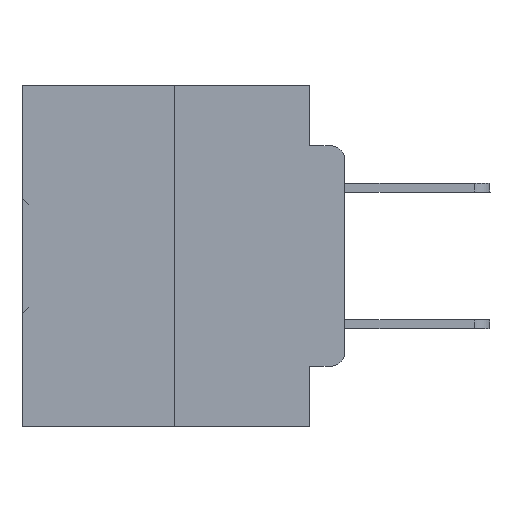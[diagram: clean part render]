
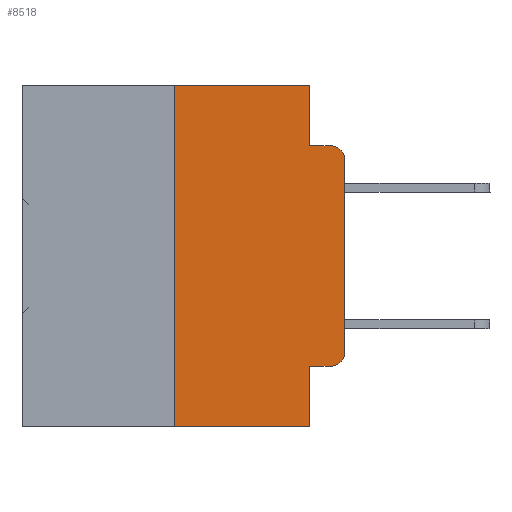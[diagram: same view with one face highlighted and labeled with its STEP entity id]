
A CAD part, left-side view. The second image highlights one B-rep face of the part: STEP entity #8518.
In plain terms, the highlighted planar face has unit normal (-1, 0, 0).
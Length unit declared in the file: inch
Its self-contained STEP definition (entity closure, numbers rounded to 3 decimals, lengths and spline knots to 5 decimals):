
#168 = DIRECTION ( 'NONE',  ( 0., -1., 0. ) ) ;
#221 = CARTESIAN_POINT ( 'NONE',  ( 0., 0.051, 0. ) ) ;
#1154 = AXIS2_PLACEMENT_3D ( 'NONE', #27815, #10689, #30720 ) ;
#1772 = FACE_OUTER_BOUND ( 'NONE', #28075, .T. ) ;
#1919 = AXIS2_PLACEMENT_3D ( 'NONE', #8920, #28961, #11852 ) ;
#1963 = DIRECTION ( 'NONE',  ( 0., -1., 0. ) ) ;
#2225 = LINE ( 'NONE', #2655, #15965 ) ;
#2399 = VERTEX_POINT ( 'NONE', #5761 ) ;
#2655 = CARTESIAN_POINT ( 'NONE',  ( 0., 0.051, 0. ) ) ;
#3067 = CARTESIAN_POINT ( 'NONE',  ( 0., 0.051, -0.0885 ) ) ;
#3183 = ORIENTED_EDGE ( 'NONE', *, *, #33127, .T. ) ;
#3220 = ORIENTED_EDGE ( 'NONE', *, *, #17807, .F. ) ;
#5761 = CARTESIAN_POINT ( 'NONE',  ( 0., 0.051, -0.5 ) ) ;
#6029 = DIRECTION ( 'NONE',  ( 0., -1., 0. ) ) ;
#6325 = VERTEX_POINT ( 'NONE', #15521 ) ;
#6991 = CARTESIAN_POINT ( 'NONE',  ( 0., 0.02, -0.4115 ) ) ;
#7839 = CARTESIAN_POINT ( 'NONE',  ( 0., 0.02, -0.0885 ) ) ;
#8230 = ORIENTED_EDGE ( 'NONE', *, *, #35025, .T. ) ;
#8272 = ORIENTED_EDGE ( 'NONE', *, *, #25946, .T. ) ;
#8518 = ADVANCED_FACE ( 'NONE', ( #1772 ), #9588, .F. ) ;
#8718 = VERTEX_POINT ( 'NONE', #33350 ) ;
#8744 = VERTEX_POINT ( 'NONE', #24830 ) ;
#8920 = CARTESIAN_POINT ( 'NONE',  ( 0., 0.02, -0.3915 ) ) ;
#9456 = CARTESIAN_POINT ( 'NONE',  ( 0., 0.473, 0. ) ) ;
#9588 = PLANE ( 'NONE',  #14633 ) ;
#10093 = DIRECTION ( 'NONE',  ( 0., 0., 1. ) ) ;
#10561 = VECTOR ( 'NONE', #32579, 39.37008 ) ;
#10689 = DIRECTION ( 'NONE',  ( -1., 0., 0. ) ) ;
#11392 = ORIENTED_EDGE ( 'NONE', *, *, #19988, .F. ) ;
#11852 = DIRECTION ( 'NONE',  ( 0., 0., -1. ) ) ;
#12070 = EDGE_CURVE ( 'NONE', #31170, #8718, #30897, .T. ) ;
#12527 = DIRECTION ( 'NONE',  ( 1., 0., 0. ) ) ;
#13017 = VERTEX_POINT ( 'NONE', #7839 ) ;
#13062 = LINE ( 'NONE', #25923, #19697 ) ;
#14633 = AXIS2_PLACEMENT_3D ( 'NONE', #9456, #12527, #32483 ) ;
#14905 = LINE ( 'NONE', #19359, #22471 ) ;
#15216 = CARTESIAN_POINT ( 'NONE',  ( 0., 0.473, 0. ) ) ;
#15521 = CARTESIAN_POINT ( 'NONE',  ( 0., 0.25, 0. ) ) ;
#15937 = EDGE_CURVE ( 'NONE', #8744, #31170, #13062, .T. ) ;
#15965 = VECTOR ( 'NONE', #34395, 39.37008 ) ;
#16024 = ORIENTED_EDGE ( 'NONE', *, *, #15937, .T. ) ;
#16224 = DIRECTION ( 'NONE',  ( 0., 0., 1. ) ) ;
#17807 = EDGE_CURVE ( 'NONE', #8744, #2399, #25761, .T. ) ;
#18100 = LINE ( 'NONE', #21829, #32390 ) ;
#18332 = CARTESIAN_POINT ( 'NONE',  ( 0., 0.051, 0. ) ) ;
#18476 = VERTEX_POINT ( 'NONE', #21540 ) ;
#18513 = LINE ( 'NONE', #15216, #32825 ) ;
#18665 = ORIENTED_EDGE ( 'NONE', *, *, #23530, .F. ) ;
#18763 = VECTOR ( 'NONE', #6029, 39.37008 ) ;
#19359 = CARTESIAN_POINT ( 'NONE',  ( 0., 0.473, -0.5 ) ) ;
#19697 = VECTOR ( 'NONE', #168, 39.37008 ) ;
#19988 = EDGE_CURVE ( 'NONE', #6325, #28095, #18513, .T. ) ;
#21540 = CARTESIAN_POINT ( 'NONE',  ( 0., 0.051, -0.0885 ) ) ;
#21829 = CARTESIAN_POINT ( 'NONE',  ( 0., 0., 0. ) ) ;
#22471 = VECTOR ( 'NONE', #1963, 39.37008 ) ;
#23530 = EDGE_CURVE ( 'NONE', #30378, #6325, #35720, .T. ) ;
#23996 = ORIENTED_EDGE ( 'NONE', *, *, #12070, .T. ) ;
#24830 = CARTESIAN_POINT ( 'NONE',  ( 0., 0.051, -0.4115 ) ) ;
#25452 = EDGE_CURVE ( 'NONE', #28095, #18476, #2225, .T. ) ;
#25464 = LINE ( 'NONE', #3067, #18763 ) ;
#25761 = LINE ( 'NONE', #18332, #10561 ) ;
#25923 = CARTESIAN_POINT ( 'NONE',  ( 0., 0.051, -0.4115 ) ) ;
#25946 = EDGE_CURVE ( 'NONE', #30378, #2399, #14905, .T. ) ;
#26724 = CIRCLE ( 'NONE', #1154, 0.02 ) ;
#27371 = EDGE_CURVE ( 'NONE', #18476, #13017, #25464, .T. ) ;
#27815 = CARTESIAN_POINT ( 'NONE',  ( 0., 0.02, -0.1085 ) ) ;
#28075 = EDGE_LOOP ( 'NONE', ( #8230, #3183, #31140, #34683, #11392, #18665, #8272, #3220, #16024, #23996 ) ) ;
#28095 = VERTEX_POINT ( 'NONE', #221 ) ;
#28961 = DIRECTION ( 'NONE',  ( -1., 0., 0. ) ) ;
#29448 = DIRECTION ( 'NONE',  ( 0., -1., 0. ) ) ;
#30116 = CARTESIAN_POINT ( 'NONE',  ( 0., 0.25, 0. ) ) ;
#30260 = CARTESIAN_POINT ( 'NONE',  ( 0., 0., -0.1085 ) ) ;
#30378 = VERTEX_POINT ( 'NONE', #35355 ) ;
#30720 = DIRECTION ( 'NONE',  ( 0., 0., -1. ) ) ;
#30897 = CIRCLE ( 'NONE', #1919, 0.02 ) ;
#31140 = ORIENTED_EDGE ( 'NONE', *, *, #27371, .F. ) ;
#31170 = VERTEX_POINT ( 'NONE', #6991 ) ;
#32390 = VECTOR ( 'NONE', #16224, 39.37008 ) ;
#32483 = DIRECTION ( 'NONE',  ( 0., 0., -1. ) ) ;
#32579 = DIRECTION ( 'NONE',  ( 0., 0., -1. ) ) ;
#32825 = VECTOR ( 'NONE', #29448, 39.37008 ) ;
#33127 = EDGE_CURVE ( 'NONE', #36151, #13017, #26724, .T. ) ;
#33350 = CARTESIAN_POINT ( 'NONE',  ( 0., 0., -0.3915 ) ) ;
#33940 = VECTOR ( 'NONE', #10093, 39.37008 ) ;
#34395 = DIRECTION ( 'NONE',  ( 0., 0., -1. ) ) ;
#34683 = ORIENTED_EDGE ( 'NONE', *, *, #25452, .F. ) ;
#35025 = EDGE_CURVE ( 'NONE', #8718, #36151, #18100, .T. ) ;
#35355 = CARTESIAN_POINT ( 'NONE',  ( 0., 0.25, -0.5 ) ) ;
#35720 = LINE ( 'NONE', #30116, #33940 ) ;
#36151 = VERTEX_POINT ( 'NONE', #30260 ) ;
